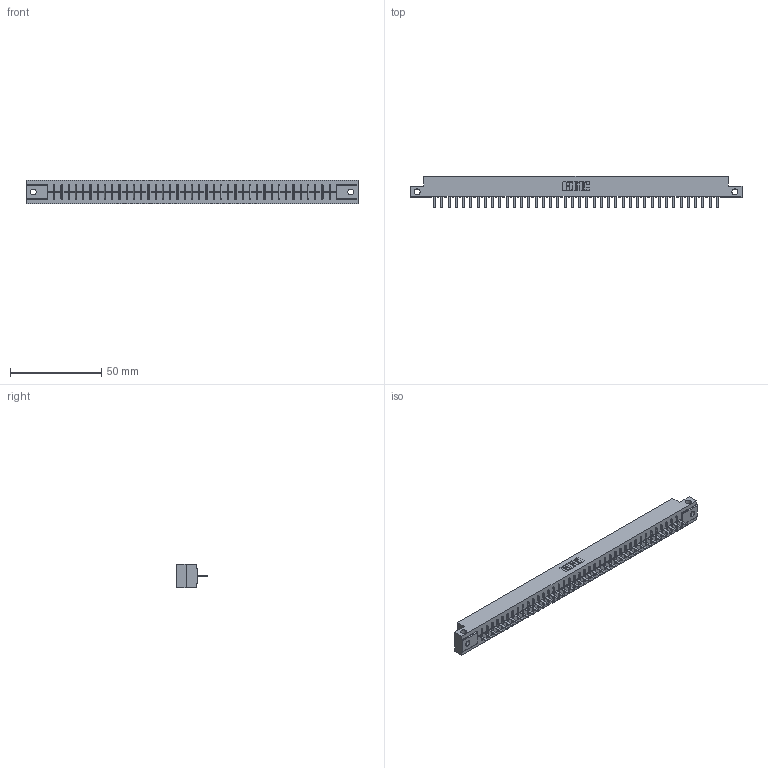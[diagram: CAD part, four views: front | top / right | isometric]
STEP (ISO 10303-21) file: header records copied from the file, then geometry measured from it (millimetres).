
FILE_DESCRIPTION (( 'STEP AP203' ), '1' );
FILE_NAME ('356-040-520-112.STEP', '2020-09-20T23:06:46', ( '' ), ( '' ), 'SwSTEP 2.0', 'SolidWorks 2020', '' );
FILE_SCHEMA (( 'CONFIG_CONTROL_DESIGN' ));
Length unit declared in the file: inch
Products named in the file (3): 306 Part_.128 Dia; 356-040-520-112; 306-290-001_120
Assembly tree (41 placements, depth 2):
  356-040-520-112
    306 Part_.128 Dia
    306-290-001_120  x40
Bounding box: 181.51 x 17.12 x 12.7 mm (x, y, z)
Volume: 19858.4 mm3; surface area: 20415.4 mm2
Topology: 41 solids, 41 shells, 2928 faces, 8232 edges, 5268 vertices
Faces by surface type: plane 1948, cylinder 820, sphere 160
Entity records: 37923 total; most frequent: CARTESIAN_POINT 6415, ORIENTED_EDGE 6316, DIRECTION 6264, EDGE_CURVE 3158, LINE 2454, VECTOR 2454, VERTEX_POINT 1992, AXIS2_PLACEMENT_3D 1905
